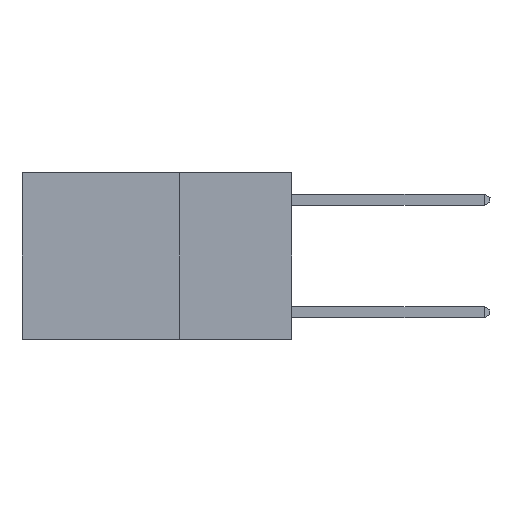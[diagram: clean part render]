
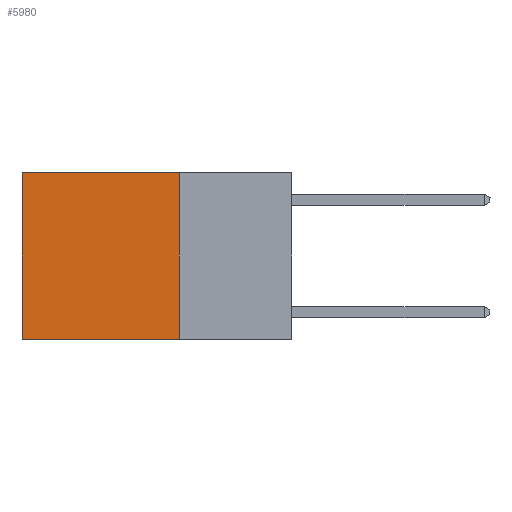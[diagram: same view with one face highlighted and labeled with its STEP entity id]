
A CAD part, left-side view. The second image highlights one B-rep face of the part: STEP entity #5980.
In plain terms, the highlighted planar face has unit normal (-1, 0, 0).
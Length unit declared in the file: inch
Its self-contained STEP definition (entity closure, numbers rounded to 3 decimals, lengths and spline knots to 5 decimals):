
#280 = CARTESIAN_POINT ( 'NONE',  ( 0.2625, 0.6, -0.37 ) ) ;
#373 = CARTESIAN_POINT ( 'NONE',  ( 0.2625, 0.25, -0.37 ) ) ;
#423 = VECTOR ( 'NONE', #5486, 39.37008 ) ;
#501 = CARTESIAN_POINT ( 'NONE',  ( 0.2625, 0.25, -0.37 ) ) ;
#622 = VERTEX_POINT ( 'NONE', #373 ) ;
#1176 = LINE ( 'NONE', #15350, #4132 ) ;
#1225 = CARTESIAN_POINT ( 'NONE',  ( 0.2625, 0.25, 0. ) ) ;
#2170 = AXIS2_PLACEMENT_3D ( 'NONE', #1225, #2515, #10961 ) ;
#2327 = DIRECTION ( 'NONE',  ( 0., 0., -1. ) ) ;
#2515 = DIRECTION ( 'NONE',  ( 1., 0., 0. ) ) ;
#2851 = EDGE_CURVE ( 'NONE', #7198, #622, #7841, .T. ) ;
#3086 = VERTEX_POINT ( 'NONE', #280 ) ;
#4132 = VECTOR ( 'NONE', #6976, 39.37008 ) ;
#4632 = DIRECTION ( 'NONE',  ( 0., 0., -1. ) ) ;
#5486 = DIRECTION ( 'NONE',  ( 0., 1., 0. ) ) ;
#5518 = ORIENTED_EDGE ( 'NONE', *, *, #2851, .F. ) ;
#5980 = ADVANCED_FACE ( 'NONE', ( #6025 ), #8543, .F. ) ;
#6019 = EDGE_LOOP ( 'NONE', ( #7484, #11284, #5518, #6205 ) ) ;
#6025 = FACE_OUTER_BOUND ( 'NONE', #6019, .T. ) ;
#6205 = ORIENTED_EDGE ( 'NONE', *, *, #7706, .T. ) ;
#6976 = DIRECTION ( 'NONE',  ( 0., 1., 0. ) ) ;
#7085 = CARTESIAN_POINT ( 'NONE',  ( 0.2625, 0.25, 0. ) ) ;
#7198 = VERTEX_POINT ( 'NONE', #7085 ) ;
#7461 = VECTOR ( 'NONE', #2327, 39.37008 ) ;
#7484 = ORIENTED_EDGE ( 'NONE', *, *, #8306, .T. ) ;
#7706 = EDGE_CURVE ( 'NONE', #7198, #12012, #1176, .T. ) ;
#7841 = LINE ( 'NONE', #11982, #7461 ) ;
#8306 = EDGE_CURVE ( 'NONE', #12012, #3086, #11443, .T. ) ;
#8543 = PLANE ( 'NONE',  #2170 ) ;
#10085 = EDGE_CURVE ( 'NONE', #622, #3086, #10155, .T. ) ;
#10155 = LINE ( 'NONE', #501, #423 ) ;
#10961 = DIRECTION ( 'NONE',  ( 0., 0., -1. ) ) ;
#11058 = VECTOR ( 'NONE', #4632, 39.37008 ) ;
#11284 = ORIENTED_EDGE ( 'NONE', *, *, #10085, .F. ) ;
#11443 = LINE ( 'NONE', #13040, #11058 ) ;
#11646 = CARTESIAN_POINT ( 'NONE',  ( 0.2625, 0.6, 0. ) ) ;
#11982 = CARTESIAN_POINT ( 'NONE',  ( 0.2625, 0.25, 0. ) ) ;
#12012 = VERTEX_POINT ( 'NONE', #11646 ) ;
#13040 = CARTESIAN_POINT ( 'NONE',  ( 0.2625, 0.6, 0. ) ) ;
#15350 = CARTESIAN_POINT ( 'NONE',  ( 0.2625, 0.25, 0. ) ) ;
